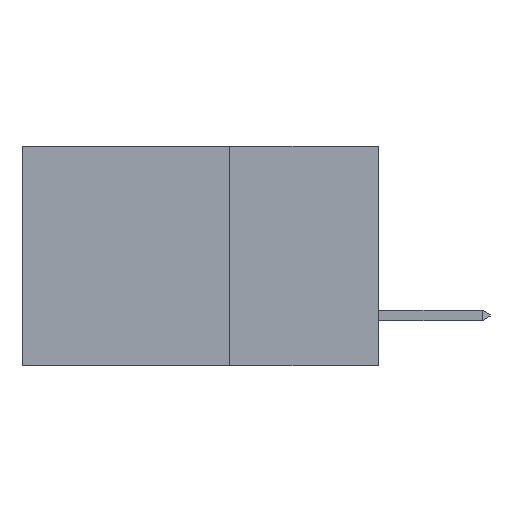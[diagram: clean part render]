
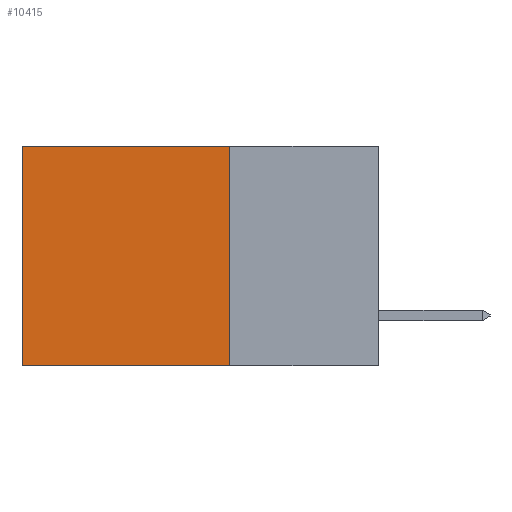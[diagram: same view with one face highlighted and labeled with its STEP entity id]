
A CAD part, left-side view. The second image highlights one B-rep face of the part: STEP entity #10415.
In plain terms, the highlighted planar face has unit normal (-1, 0, 0).
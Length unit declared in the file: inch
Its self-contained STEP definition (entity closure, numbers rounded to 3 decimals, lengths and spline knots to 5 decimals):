
#143 = CARTESIAN_POINT ( 'NONE',  ( 0.298, 0.6, 0. ) ) ;
#355 = VECTOR ( 'NONE', #22399, 39.37008 ) ;
#965 = VECTOR ( 'NONE', #9260, 39.37008 ) ;
#2501 = VECTOR ( 'NONE', #5930, 39.37008 ) ;
#3639 = VERTEX_POINT ( 'NONE', #20624 ) ;
#4551 = CARTESIAN_POINT ( 'NONE',  ( 0.298, 0.25, 0. ) ) ;
#5364 = DIRECTION ( 'NONE',  ( 0., 0., -1. ) ) ;
#5930 = DIRECTION ( 'NONE',  ( 0., 1., 0. ) ) ;
#6113 = VERTEX_POINT ( 'NONE', #143 ) ;
#7329 = CARTESIAN_POINT ( 'NONE',  ( 0.298, 0.6, 0. ) ) ;
#7562 = LINE ( 'NONE', #22994, #2501 ) ;
#9102 = PLANE ( 'NONE',  #17998 ) ;
#9260 = DIRECTION ( 'NONE',  ( 0., 0., -1. ) ) ;
#10205 = DIRECTION ( 'NONE',  ( 0., 1., 0. ) ) ;
#10226 = VECTOR ( 'NONE', #10205, 39.37008 ) ;
#10415 = ADVANCED_FACE ( 'NONE', ( #20891 ), #9102, .F. ) ;
#10485 = EDGE_LOOP ( 'NONE', ( #18340, #15732, #23458, #24190 ) ) ;
#11177 = LINE ( 'NONE', #7329, #965 ) ;
#11391 = CARTESIAN_POINT ( 'NONE',  ( 0.298, 0.6, -0.37 ) ) ;
#11704 = VERTEX_POINT ( 'NONE', #11391 ) ;
#14216 = EDGE_CURVE ( 'NONE', #6113, #11704, #11177, .T. ) ;
#14395 = EDGE_CURVE ( 'NONE', #16161, #11704, #7562, .T. ) ;
#14898 = EDGE_CURVE ( 'NONE', #3639, #6113, #20341, .T. ) ;
#14946 = CARTESIAN_POINT ( 'NONE',  ( 0.298, 0.25, 0. ) ) ;
#15732 = ORIENTED_EDGE ( 'NONE', *, *, #14395, .F. ) ;
#16161 = VERTEX_POINT ( 'NONE', #18079 ) ;
#16821 = DIRECTION ( 'NONE',  ( 1., 0., 0. ) ) ;
#17998 = AXIS2_PLACEMENT_3D ( 'NONE', #14946, #16821, #5364 ) ;
#18079 = CARTESIAN_POINT ( 'NONE',  ( 0.298, 0.25, -0.37 ) ) ;
#18340 = ORIENTED_EDGE ( 'NONE', *, *, #14216, .T. ) ;
#20068 = LINE ( 'NONE', #20535, #355 ) ;
#20341 = LINE ( 'NONE', #4551, #10226 ) ;
#20535 = CARTESIAN_POINT ( 'NONE',  ( 0.298, 0.25, 0. ) ) ;
#20624 = CARTESIAN_POINT ( 'NONE',  ( 0.298, 0.25, 0. ) ) ;
#20891 = FACE_OUTER_BOUND ( 'NONE', #10485, .T. ) ;
#21074 = EDGE_CURVE ( 'NONE', #3639, #16161, #20068, .T. ) ;
#22399 = DIRECTION ( 'NONE',  ( 0., 0., -1. ) ) ;
#22994 = CARTESIAN_POINT ( 'NONE',  ( 0.298, 0.25, -0.37 ) ) ;
#23458 = ORIENTED_EDGE ( 'NONE', *, *, #21074, .F. ) ;
#24190 = ORIENTED_EDGE ( 'NONE', *, *, #14898, .T. ) ;
